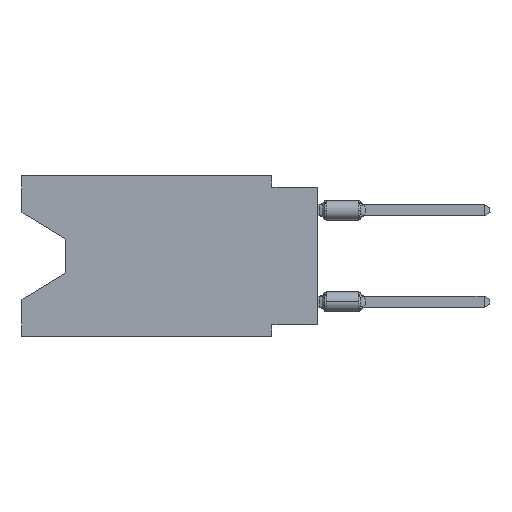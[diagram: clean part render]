
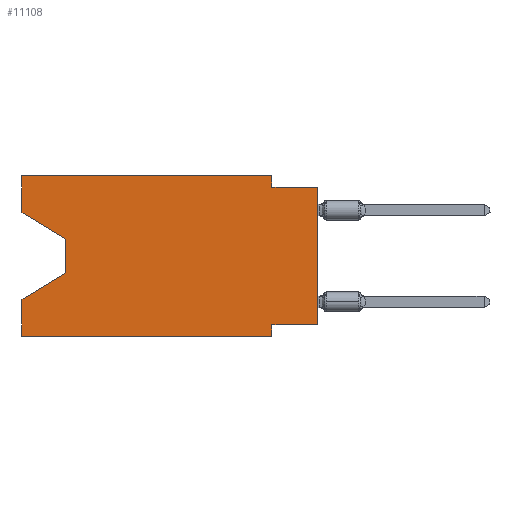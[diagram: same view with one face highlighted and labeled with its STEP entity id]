
A CAD part, left-side view. The second image highlights one B-rep face of the part: STEP entity #11108.
In plain terms, the highlighted planar face has unit normal (-1, 0, 0).
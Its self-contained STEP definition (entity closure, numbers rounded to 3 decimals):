
#262 = DIRECTION ( 'NONE',  ( 0., 0., 1. ) ) ;
#1269 = CARTESIAN_POINT ( 'NONE',  ( 0., 2.54, -8.89 ) ) ;
#1678 = DIRECTION ( 'NONE',  ( 0., 0., -1. ) ) ;
#2202 = LINE ( 'NONE', #22048, #9652 ) ;
#2720 = LINE ( 'NONE', #31666, #4946 ) ;
#3363 = VERTEX_POINT ( 'NONE', #24829 ) ;
#3744 = DIRECTION ( 'NONE',  ( 0., -0.855, -0.519 ) ) ;
#3781 = PLANE ( 'NONE',  #32533 ) ;
#3897 = ORIENTED_EDGE ( 'NONE', *, *, #5227, .F. ) ;
#4339 = CARTESIAN_POINT ( 'NONE',  ( 0., 2.54, -8.89 ) ) ;
#4946 = VECTOR ( 'NONE', #14016, 1000. ) ;
#4999 = DIRECTION ( 'NONE',  ( 0., 0., 1. ) ) ;
#5227 = EDGE_CURVE ( 'NONE', #33805, #26306, #15468, .T. ) ;
#6268 = VERTEX_POINT ( 'NONE', #33889 ) ;
#6519 = LINE ( 'NONE', #32319, #11214 ) ;
#7054 = CARTESIAN_POINT ( 'NONE',  ( 0., 16.383, -6.852 ) ) ;
#7114 = DIRECTION ( 'NONE',  ( 0., 0., 1. ) ) ;
#7169 = LINE ( 'NONE', #1269, #25090 ) ;
#7381 = ORIENTED_EDGE ( 'NONE', *, *, #33512, .F. ) ;
#7393 = ORIENTED_EDGE ( 'NONE', *, *, #23470, .T. ) ;
#8243 = EDGE_CURVE ( 'NONE', #22889, #16766, #28651, .T. ) ;
#8260 = VERTEX_POINT ( 'NONE', #20852 ) ;
#8956 = CARTESIAN_POINT ( 'NONE',  ( 0., 16.383, 0. ) ) ;
#9291 = LINE ( 'NONE', #31960, #34726 ) ;
#9345 = CARTESIAN_POINT ( 'NONE',  ( 0., 13.97, -3.505 ) ) ;
#9652 = VECTOR ( 'NONE', #35807, 1000. ) ;
#9839 = DIRECTION ( 'NONE',  ( 0., -1., 0. ) ) ;
#10145 = ORIENTED_EDGE ( 'NONE', *, *, #16899, .T. ) ;
#10548 = LINE ( 'NONE', #30236, #34650 ) ;
#10695 = VERTEX_POINT ( 'NONE', #30289 ) ;
#11108 = ADVANCED_FACE ( 'NONE', ( #29198 ), #3781, .F. ) ;
#11214 = VECTOR ( 'NONE', #3744, 1000. ) ;
#12250 = EDGE_LOOP ( 'NONE', ( #15704, #7393, #32894, #17560, #18149, #7381, #33259, #10145, #18883, #3897, #15763, #16854 ) ) ;
#12486 = LINE ( 'NONE', #35709, #13287 ) ;
#12743 = DIRECTION ( 'NONE',  ( 0., 0., -1. ) ) ;
#13287 = VECTOR ( 'NONE', #29575, 1000. ) ;
#14016 = DIRECTION ( 'NONE',  ( 0., 0.855, -0.519 ) ) ;
#14024 = CARTESIAN_POINT ( 'NONE',  ( 0., 0., 0. ) ) ;
#14255 = LINE ( 'NONE', #14024, #21357 ) ;
#15468 = LINE ( 'NONE', #26613, #24486 ) ;
#15654 = CARTESIAN_POINT ( 'NONE',  ( 0., 16.383, 0. ) ) ;
#15704 = ORIENTED_EDGE ( 'NONE', *, *, #16650, .T. ) ;
#15763 = ORIENTED_EDGE ( 'NONE', *, *, #26753, .F. ) ;
#16469 = CARTESIAN_POINT ( 'NONE',  ( 0., 2.54, -0.635 ) ) ;
#16650 = EDGE_CURVE ( 'NONE', #6268, #28826, #6519, .T. ) ;
#16766 = VERTEX_POINT ( 'NONE', #7054 ) ;
#16854 = ORIENTED_EDGE ( 'NONE', *, *, #31189, .F. ) ;
#16899 = EDGE_CURVE ( 'NONE', #21433, #3363, #14255, .T. ) ;
#17560 = ORIENTED_EDGE ( 'NONE', *, *, #8243, .F. ) ;
#17917 = EDGE_CURVE ( 'NONE', #22889, #28771, #9291, .T. ) ;
#18149 = ORIENTED_EDGE ( 'NONE', *, *, #17917, .T. ) ;
#18883 = ORIENTED_EDGE ( 'NONE', *, *, #35047, .F. ) ;
#19167 = VECTOR ( 'NONE', #7114, 1000. ) ;
#19177 = CARTESIAN_POINT ( 'NONE',  ( 0., 0., -8.255 ) ) ;
#19259 = LINE ( 'NONE', #28152, #21655 ) ;
#20339 = CARTESIAN_POINT ( 'NONE',  ( 0., 2.54, 0. ) ) ;
#20852 = CARTESIAN_POINT ( 'NONE',  ( 0., 13.97, -5.385 ) ) ;
#21357 = VECTOR ( 'NONE', #4999, 1000. ) ;
#21433 = VERTEX_POINT ( 'NONE', #19177 ) ;
#21655 = VECTOR ( 'NONE', #36527, 1000. ) ;
#22048 = CARTESIAN_POINT ( 'NONE',  ( 0., 0., -8.255 ) ) ;
#22348 = EDGE_CURVE ( 'NONE', #21433, #10695, #2202, .T. ) ;
#22889 = VERTEX_POINT ( 'NONE', #23442 ) ;
#23263 = DIRECTION ( 'NONE',  ( 1., 0., 0. ) ) ;
#23442 = CARTESIAN_POINT ( 'NONE',  ( 0., 16.383, -8.89 ) ) ;
#23470 = EDGE_CURVE ( 'NONE', #28826, #8260, #10548, .T. ) ;
#24486 = VECTOR ( 'NONE', #32382, 1000. ) ;
#24829 = CARTESIAN_POINT ( 'NONE',  ( 0., 0., -0.635 ) ) ;
#25090 = VECTOR ( 'NONE', #12743, 1000. ) ;
#25678 = CARTESIAN_POINT ( 'NONE',  ( 0., 16.383, 0. ) ) ;
#25925 = LINE ( 'NONE', #15654, #19167 ) ;
#26306 = VERTEX_POINT ( 'NONE', #16469 ) ;
#26613 = CARTESIAN_POINT ( 'NONE',  ( 0., 2.54, 0. ) ) ;
#26753 = EDGE_CURVE ( 'NONE', #35240, #33805, #19259, .T. ) ;
#28152 = CARTESIAN_POINT ( 'NONE',  ( 0., 16.383, 0. ) ) ;
#28651 = LINE ( 'NONE', #25678, #28783 ) ;
#28771 = VERTEX_POINT ( 'NONE', #4339 ) ;
#28783 = VECTOR ( 'NONE', #262, 1000. ) ;
#28826 = VERTEX_POINT ( 'NONE', #9345 ) ;
#29198 = FACE_OUTER_BOUND ( 'NONE', #12250, .T. ) ;
#29575 = DIRECTION ( 'NONE',  ( 0., -1., 0. ) ) ;
#30236 = CARTESIAN_POINT ( 'NONE',  ( 0., 13.97, -3.505 ) ) ;
#30289 = CARTESIAN_POINT ( 'NONE',  ( 0., 2.54, -8.255 ) ) ;
#31189 = EDGE_CURVE ( 'NONE', #6268, #35240, #25925, .T. ) ;
#31628 = DIRECTION ( 'NONE',  ( 0., 0., -1. ) ) ;
#31666 = CARTESIAN_POINT ( 'NONE',  ( 0., 13.97, -5.385 ) ) ;
#31960 = CARTESIAN_POINT ( 'NONE',  ( 0., 16.383, -8.89 ) ) ;
#32319 = CARTESIAN_POINT ( 'NONE',  ( 0., 16.383, -2.038 ) ) ;
#32382 = DIRECTION ( 'NONE',  ( 0., 0., -1. ) ) ;
#32533 = AXIS2_PLACEMENT_3D ( 'NONE', #8956, #23263, #31628 ) ;
#32894 = ORIENTED_EDGE ( 'NONE', *, *, #33870, .T. ) ;
#33259 = ORIENTED_EDGE ( 'NONE', *, *, #22348, .F. ) ;
#33512 = EDGE_CURVE ( 'NONE', #10695, #28771, #7169, .T. ) ;
#33805 = VERTEX_POINT ( 'NONE', #20339 ) ;
#33870 = EDGE_CURVE ( 'NONE', #8260, #16766, #2720, .T. ) ;
#33889 = CARTESIAN_POINT ( 'NONE',  ( 0., 16.383, -2.038 ) ) ;
#34650 = VECTOR ( 'NONE', #1678, 1000. ) ;
#34726 = VECTOR ( 'NONE', #9839, 1000. ) ;
#35047 = EDGE_CURVE ( 'NONE', #26306, #3363, #12486, .T. ) ;
#35240 = VERTEX_POINT ( 'NONE', #36265 ) ;
#35709 = CARTESIAN_POINT ( 'NONE',  ( 0., 0., -0.635 ) ) ;
#35807 = DIRECTION ( 'NONE',  ( 0., 1., 0. ) ) ;
#36265 = CARTESIAN_POINT ( 'NONE',  ( 0., 16.383, 0. ) ) ;
#36527 = DIRECTION ( 'NONE',  ( 0., -1., 0. ) ) ;
